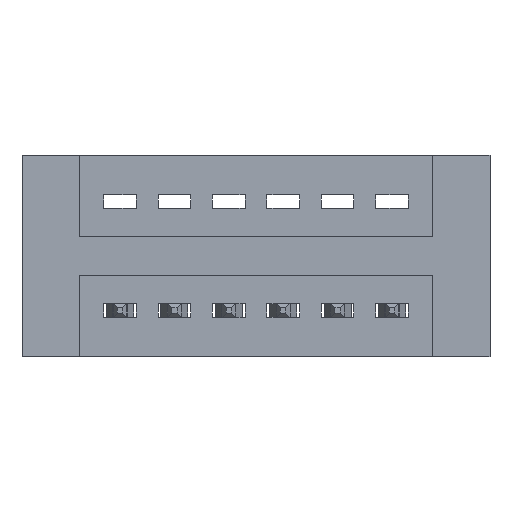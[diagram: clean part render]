
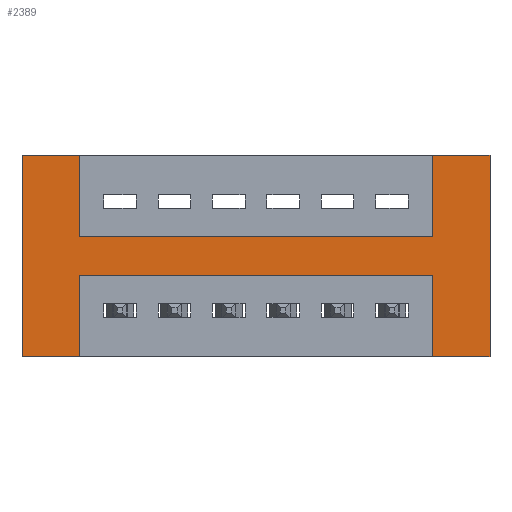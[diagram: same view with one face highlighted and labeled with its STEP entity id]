
A CAD part, front view. The second image highlights one B-rep face of the part: STEP entity #2389.
In plain terms, the highlighted planar face has unit normal (0, -1, 0).
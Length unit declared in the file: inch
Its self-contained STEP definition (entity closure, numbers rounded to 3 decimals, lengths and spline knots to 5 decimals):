
#4 = EDGE_CURVE ( 'NONE', #744, #4921, #3677, .T. ) ;
#82 = DIRECTION ( 'NONE',  ( 1., 0., 0. ) ) ;
#213 = CARTESIAN_POINT ( 'NONE',  ( 0., 0., 0. ) ) ;
#435 = VERTEX_POINT ( 'NONE', #2626 ) ;
#449 = VERTEX_POINT ( 'NONE', #7732 ) ;
#531 = LINE ( 'NONE', #3763, #4177 ) ;
#546 = DIRECTION ( 'NONE',  ( 0., 0., 1. ) ) ;
#627 = LINE ( 'NONE', #1758, #8749 ) ;
#697 = CARTESIAN_POINT ( 'NONE',  ( 0.2875, 0., -0.37 ) ) ;
#720 = LINE ( 'NONE', #3603, #4143 ) ;
#744 = VERTEX_POINT ( 'NONE', #2135 ) ;
#778 = EDGE_CURVE ( 'NONE', #1935, #6351, #6808, .T. ) ;
#871 = DIRECTION ( 'NONE',  ( -1., 0., 0. ) ) ;
#894 = EDGE_CURVE ( 'NONE', #6659, #4993, #4766, .T. ) ;
#1018 = LINE ( 'NONE', #2820, #3663 ) ;
#1084 = DIRECTION ( 'NONE',  ( 0., 0., 1. ) ) ;
#1181 = LINE ( 'NONE', #1910, #4282 ) ;
#1319 = LINE ( 'NONE', #213, #3082 ) ;
#1378 = DIRECTION ( 'NONE',  ( -1., 0., 0. ) ) ;
#1434 = CARTESIAN_POINT ( 'NONE',  ( 0.3925, 0., -0.22 ) ) ;
#1549 = CARTESIAN_POINT ( 'NONE',  ( 0.3925, 0., -0.22 ) ) ;
#1628 = VECTOR ( 'NONE', #8996, 39.37008 ) ;
#1758 = CARTESIAN_POINT ( 'NONE',  ( 0., 0., 0. ) ) ;
#1803 = ORIENTED_EDGE ( 'NONE', *, *, #3213, .F. ) ;
#1889 = CARTESIAN_POINT ( 'NONE',  ( 1.0425, 0., -0.37 ) ) ;
#1910 = CARTESIAN_POINT ( 'NONE',  ( 1.0425, 0., 0. ) ) ;
#1935 = VERTEX_POINT ( 'NONE', #7095 ) ;
#1948 = EDGE_CURVE ( 'NONE', #435, #449, #1018, .T. ) ;
#1977 = ORIENTED_EDGE ( 'NONE', *, *, #5489, .T. ) ;
#2109 = LINE ( 'NONE', #7112, #6925 ) ;
#2135 = CARTESIAN_POINT ( 'NONE',  ( 0.3925, 0., -0.37 ) ) ;
#2201 = DIRECTION ( 'NONE',  ( -1., 0., 0. ) ) ;
#2202 = AXIS2_PLACEMENT_3D ( 'NONE', #6162, #6873, #2648 ) ;
#2283 = ORIENTED_EDGE ( 'NONE', *, *, #4, .F. ) ;
#2311 = VERTEX_POINT ( 'NONE', #5279 ) ;
#2350 = VERTEX_POINT ( 'NONE', #2501 ) ;
#2389 = ADVANCED_FACE ( 'NONE', ( #8926 ), #2594, .T. ) ;
#2462 = DIRECTION ( 'NONE',  ( 0., 0., -1. ) ) ;
#2501 = CARTESIAN_POINT ( 'NONE',  ( 1.0425, 0., 0. ) ) ;
#2594 = PLANE ( 'NONE',  #2202 ) ;
#2626 = CARTESIAN_POINT ( 'NONE',  ( 0.3925, 0., 0. ) ) ;
#2648 = DIRECTION ( 'NONE',  ( 0., 0., -1. ) ) ;
#2820 = CARTESIAN_POINT ( 'NONE',  ( 0.3925, 0., 0. ) ) ;
#2900 = ORIENTED_EDGE ( 'NONE', *, *, #8888, .F. ) ;
#2991 = ORIENTED_EDGE ( 'NONE', *, *, #1948, .F. ) ;
#3082 = VECTOR ( 'NONE', #7890, 39.37008 ) ;
#3152 = CARTESIAN_POINT ( 'NONE',  ( 1.1475, 0., 0. ) ) ;
#3213 = EDGE_CURVE ( 'NONE', #3289, #6659, #5689, .T. ) ;
#3251 = DIRECTION ( 'NONE',  ( 0., 0., 1. ) ) ;
#3289 = VERTEX_POINT ( 'NONE', #3400 ) ;
#3400 = CARTESIAN_POINT ( 'NONE',  ( 1.0425, 0., -0.37 ) ) ;
#3404 = CARTESIAN_POINT ( 'NONE',  ( 0., 0., -0.37 ) ) ;
#3442 = CARTESIAN_POINT ( 'NONE',  ( 1.1475, 0., 0. ) ) ;
#3525 = DIRECTION ( 'NONE',  ( 0., 0., -1. ) ) ;
#3603 = CARTESIAN_POINT ( 'NONE',  ( 0.3925, 0., -0.15 ) ) ;
#3608 = ORIENTED_EDGE ( 'NONE', *, *, #894, .F. ) ;
#3663 = VECTOR ( 'NONE', #3525, 39.37008 ) ;
#3677 = LINE ( 'NONE', #3404, #4128 ) ;
#3733 = EDGE_CURVE ( 'NONE', #4993, #744, #531, .T. ) ;
#3763 = CARTESIAN_POINT ( 'NONE',  ( 0.3925, 0., -0.37 ) ) ;
#3795 = EDGE_CURVE ( 'NONE', #2311, #2350, #1181, .T. ) ;
#4094 = EDGE_CURVE ( 'NONE', #2350, #6351, #627, .T. ) ;
#4128 = VECTOR ( 'NONE', #2201, 39.37008 ) ;
#4143 = VECTOR ( 'NONE', #82, 39.37008 ) ;
#4177 = VECTOR ( 'NONE', #2462, 39.37008 ) ;
#4282 = VECTOR ( 'NONE', #1084, 39.37008 ) ;
#4385 = ORIENTED_EDGE ( 'NONE', *, *, #3733, .F. ) ;
#4442 = VECTOR ( 'NONE', #3251, 39.37008 ) ;
#4766 = LINE ( 'NONE', #1434, #6175 ) ;
#4921 = VERTEX_POINT ( 'NONE', #697 ) ;
#4970 = CARTESIAN_POINT ( 'NONE',  ( 1.0425, 0., -0.22 ) ) ;
#4993 = VERTEX_POINT ( 'NONE', #1549 ) ;
#5128 = EDGE_CURVE ( 'NONE', #1935, #3289, #2109, .T. ) ;
#5141 = ORIENTED_EDGE ( 'NONE', *, *, #3795, .F. ) ;
#5279 = CARTESIAN_POINT ( 'NONE',  ( 1.0425, 0., -0.15 ) ) ;
#5440 = VERTEX_POINT ( 'NONE', #9098 ) ;
#5474 = VECTOR ( 'NONE', #546, 39.37008 ) ;
#5489 = EDGE_CURVE ( 'NONE', #5440, #4921, #7236, .T. ) ;
#5539 = ORIENTED_EDGE ( 'NONE', *, *, #5128, .F. ) ;
#5560 = CARTESIAN_POINT ( 'NONE',  ( 0.2875, 0., 0. ) ) ;
#5689 = LINE ( 'NONE', #1889, #5474 ) ;
#5981 = DIRECTION ( 'NONE',  ( 1., 0., 0. ) ) ;
#6023 = ORIENTED_EDGE ( 'NONE', *, *, #778, .T. ) ;
#6162 = CARTESIAN_POINT ( 'NONE',  ( 0., 0., -0.37 ) ) ;
#6175 = VECTOR ( 'NONE', #1378, 39.37008 ) ;
#6351 = VERTEX_POINT ( 'NONE', #3442 ) ;
#6659 = VERTEX_POINT ( 'NONE', #4970 ) ;
#6808 = LINE ( 'NONE', #3152, #4442 ) ;
#6827 = ORIENTED_EDGE ( 'NONE', *, *, #7778, .F. ) ;
#6873 = DIRECTION ( 'NONE',  ( 0., -1., 0. ) ) ;
#6925 = VECTOR ( 'NONE', #871, 39.37008 ) ;
#7095 = CARTESIAN_POINT ( 'NONE',  ( 1.1475, 0., -0.37 ) ) ;
#7112 = CARTESIAN_POINT ( 'NONE',  ( 0., 0., -0.37 ) ) ;
#7176 = ORIENTED_EDGE ( 'NONE', *, *, #4094, .F. ) ;
#7236 = LINE ( 'NONE', #5560, #1628 ) ;
#7732 = CARTESIAN_POINT ( 'NONE',  ( 0.3925, 0., -0.15 ) ) ;
#7778 = EDGE_CURVE ( 'NONE', #5440, #435, #1319, .T. ) ;
#7890 = DIRECTION ( 'NONE',  ( 1., 0., 0. ) ) ;
#8392 = EDGE_LOOP ( 'NONE', ( #6023, #7176, #5141, #2900, #2991, #6827, #1977, #2283, #4385, #3608, #1803, #5539 ) ) ;
#8749 = VECTOR ( 'NONE', #5981, 39.37008 ) ;
#8888 = EDGE_CURVE ( 'NONE', #449, #2311, #720, .T. ) ;
#8926 = FACE_OUTER_BOUND ( 'NONE', #8392, .T. ) ;
#8996 = DIRECTION ( 'NONE',  ( 0., 0., -1. ) ) ;
#9098 = CARTESIAN_POINT ( 'NONE',  ( 0.2875, 0., 0. ) ) ;
